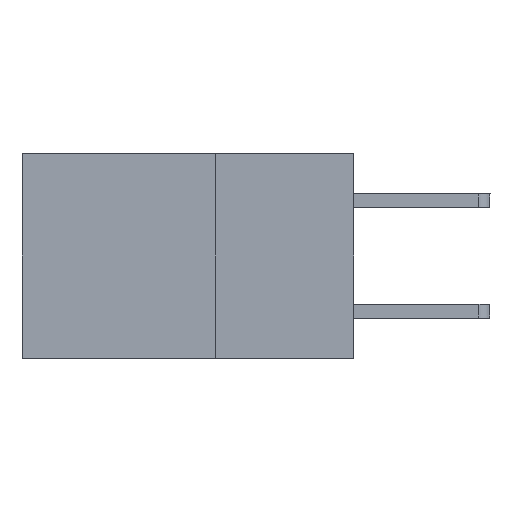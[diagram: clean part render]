
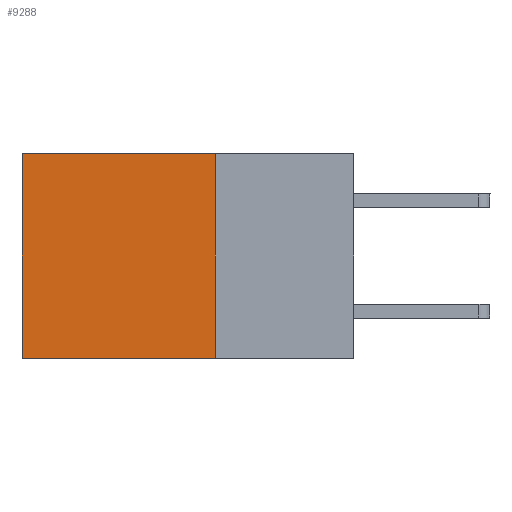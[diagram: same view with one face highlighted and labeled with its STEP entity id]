
A CAD part, left-side view. The second image highlights one B-rep face of the part: STEP entity #9288.
In plain terms, the highlighted planar face has unit normal (-1, 0, 0).
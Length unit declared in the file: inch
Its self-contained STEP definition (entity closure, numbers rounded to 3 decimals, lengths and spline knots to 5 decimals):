
#38 = VERTEX_POINT ( 'NONE', #4006 ) ;
#201 = DIRECTION ( 'NONE',  ( 0., 1., 0. ) ) ;
#420 = CARTESIAN_POINT ( 'NONE',  ( 0.2875, 0.25, -0.37 ) ) ;
#469 = EDGE_LOOP ( 'NONE', ( #4938, #4958, #5001, #5013 ) ) ;
#859 = CARTESIAN_POINT ( 'NONE',  ( 0.2875, 0.25, 0. ) ) ;
#1078 = LINE ( 'NONE', #859, #8902 ) ;
#2160 = DIRECTION ( 'NONE',  ( 0., 1., 0. ) ) ;
#2717 = DIRECTION ( 'NONE',  ( 0., 0., -1. ) ) ;
#3024 = CARTESIAN_POINT ( 'NONE',  ( 0.2875, 0.25, 0. ) ) ;
#3412 = CARTESIAN_POINT ( 'NONE',  ( 0.2875, 0.6, 0. ) ) ;
#3550 = EDGE_CURVE ( 'NONE', #5721, #5585, #6577, .T. ) ;
#3787 = EDGE_CURVE ( 'NONE', #5585, #38, #6636, .T. ) ;
#4006 = CARTESIAN_POINT ( 'NONE',  ( 0.2875, 0.6, -0.37 ) ) ;
#4236 = DIRECTION ( 'NONE',  ( 0., 0., -1. ) ) ;
#4443 = EDGE_CURVE ( 'NONE', #5721, #6159, #1078, .T. ) ;
#4580 = VECTOR ( 'NONE', #201, 39.37008 ) ;
#4776 = CARTESIAN_POINT ( 'NONE',  ( 0.2875, 0.25, 0. ) ) ;
#4938 = ORIENTED_EDGE ( 'NONE', *, *, #7720, .T. ) ;
#4958 = ORIENTED_EDGE ( 'NONE', *, *, #3787, .F. ) ;
#5001 = ORIENTED_EDGE ( 'NONE', *, *, #3550, .F. ) ;
#5013 = ORIENTED_EDGE ( 'NONE', *, *, #4443, .T. ) ;
#5207 = LINE ( 'NONE', #3412, #8972 ) ;
#5548 = DIRECTION ( 'NONE',  ( 0., 0., -1. ) ) ;
#5585 = VERTEX_POINT ( 'NONE', #8807 ) ;
#5624 = CARTESIAN_POINT ( 'NONE',  ( 0.2875, 0.6, 0. ) ) ;
#5721 = VERTEX_POINT ( 'NONE', #8049 ) ;
#6159 = VERTEX_POINT ( 'NONE', #5624 ) ;
#6577 = LINE ( 'NONE', #3024, #8238 ) ;
#6636 = LINE ( 'NONE', #420, #4580 ) ;
#7449 = AXIS2_PLACEMENT_3D ( 'NONE', #4776, #9994, #5548 ) ;
#7689 = FACE_OUTER_BOUND ( 'NONE', #469, .T. ) ;
#7720 = EDGE_CURVE ( 'NONE', #6159, #38, #5207, .T. ) ;
#8049 = CARTESIAN_POINT ( 'NONE',  ( 0.2875, 0.25, 0. ) ) ;
#8238 = VECTOR ( 'NONE', #2717, 39.37008 ) ;
#8807 = CARTESIAN_POINT ( 'NONE',  ( 0.2875, 0.25, -0.37 ) ) ;
#8902 = VECTOR ( 'NONE', #2160, 39.37008 ) ;
#8972 = VECTOR ( 'NONE', #4236, 39.37008 ) ;
#9271 = PLANE ( 'NONE',  #7449 ) ;
#9288 = ADVANCED_FACE ( 'NONE', ( #7689 ), #9271, .F. ) ;
#9994 = DIRECTION ( 'NONE',  ( 1., 0., 0. ) ) ;
